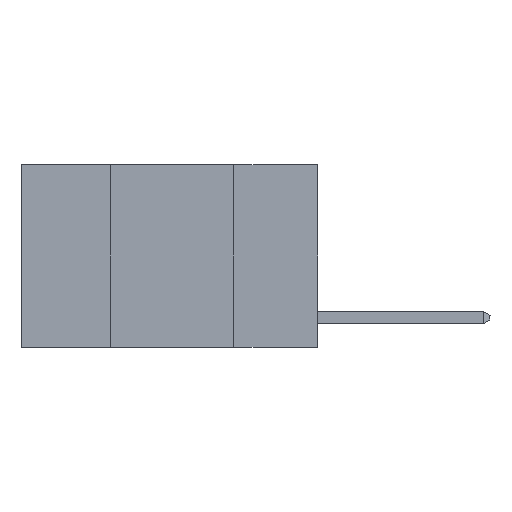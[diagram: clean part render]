
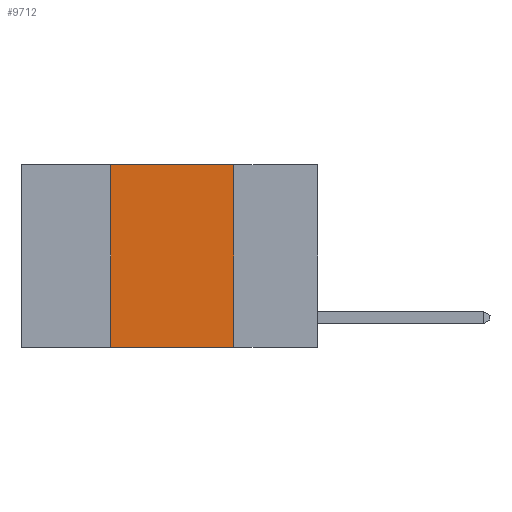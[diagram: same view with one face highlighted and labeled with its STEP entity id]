
A CAD part, left-side view. The second image highlights one B-rep face of the part: STEP entity #9712.
In plain terms, the highlighted planar face has unit normal (-1, 0, 0).
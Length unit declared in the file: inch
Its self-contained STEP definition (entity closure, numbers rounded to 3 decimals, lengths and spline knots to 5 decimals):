
#577 = VERTEX_POINT ( 'NONE', #27504 ) ;
#1308 = EDGE_LOOP ( 'NONE', ( #15396, #28139, #21154, #15783 ) ) ;
#1327 = PLANE ( 'NONE',  #26339 ) ;
#3506 = FACE_OUTER_BOUND ( 'NONE', #1308, .T. ) ;
#5315 = LINE ( 'NONE', #18918, #13460 ) ;
#5735 = DIRECTION ( 'NONE',  ( 0., 0., -1. ) ) ;
#6216 = EDGE_CURVE ( 'NONE', #27604, #577, #5315, .T. ) ;
#7080 = EDGE_CURVE ( 'NONE', #17812, #27604, #14599, .T. ) ;
#7964 = CARTESIAN_POINT ( 'NONE',  ( 0., 0.6, -0.37 ) ) ;
#9644 = CARTESIAN_POINT ( 'NONE',  ( 0., 0.42, 0. ) ) ;
#9712 = ADVANCED_FACE ( 'NONE', ( #3506 ), #1327, .F. ) ;
#10374 = CARTESIAN_POINT ( 'NONE',  ( 0., 0.17, 0. ) ) ;
#10638 = DIRECTION ( 'NONE',  ( 0., 0., 1. ) ) ;
#12337 = DIRECTION ( 'NONE',  ( 1., 0., 0. ) ) ;
#13460 = VECTOR ( 'NONE', #5735, 39.37008 ) ;
#14364 = CARTESIAN_POINT ( 'NONE',  ( 0., 0.6, 0. ) ) ;
#14599 = LINE ( 'NONE', #28044, #19313 ) ;
#14905 = LINE ( 'NONE', #7964, #25166 ) ;
#15396 = ORIENTED_EDGE ( 'NONE', *, *, #6216, .F. ) ;
#15783 = ORIENTED_EDGE ( 'NONE', *, *, #15907, .T. ) ;
#15907 = EDGE_CURVE ( 'NONE', #18676, #577, #14905, .T. ) ;
#17812 = VERTEX_POINT ( 'NONE', #9644 ) ;
#18676 = VERTEX_POINT ( 'NONE', #20527 ) ;
#18918 = CARTESIAN_POINT ( 'NONE',  ( 0., 0.17, 0. ) ) ;
#19125 = DIRECTION ( 'NONE',  ( 0., 0., -1. ) ) ;
#19313 = VECTOR ( 'NONE', #27895, 39.37008 ) ;
#20505 = VECTOR ( 'NONE', #10638, 39.37008 ) ;
#20527 = CARTESIAN_POINT ( 'NONE',  ( 0., 0.42, -0.37 ) ) ;
#20769 = EDGE_CURVE ( 'NONE', #18676, #17812, #23946, .T. ) ;
#21154 = ORIENTED_EDGE ( 'NONE', *, *, #20769, .F. ) ;
#21411 = DIRECTION ( 'NONE',  ( 0., -1., 0. ) ) ;
#21622 = CARTESIAN_POINT ( 'NONE',  ( 0., 0.42, 0. ) ) ;
#23946 = LINE ( 'NONE', #21622, #20505 ) ;
#25166 = VECTOR ( 'NONE', #21411, 39.37008 ) ;
#26339 = AXIS2_PLACEMENT_3D ( 'NONE', #14364, #12337, #19125 ) ;
#27504 = CARTESIAN_POINT ( 'NONE',  ( 0., 0.17, -0.37 ) ) ;
#27604 = VERTEX_POINT ( 'NONE', #10374 ) ;
#27895 = DIRECTION ( 'NONE',  ( 0., -1., 0. ) ) ;
#28044 = CARTESIAN_POINT ( 'NONE',  ( 0., 0.6, 0. ) ) ;
#28139 = ORIENTED_EDGE ( 'NONE', *, *, #7080, .F. ) ;
